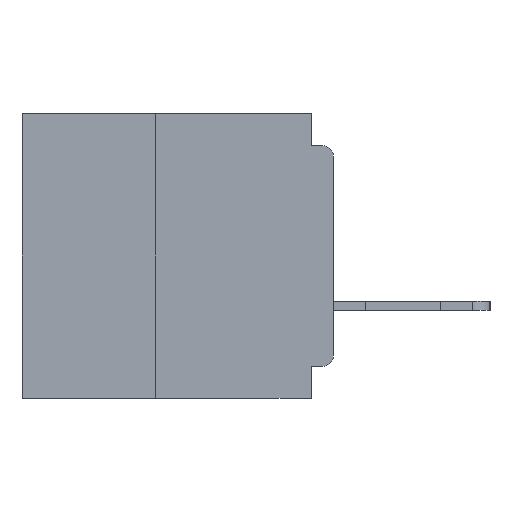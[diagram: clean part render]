
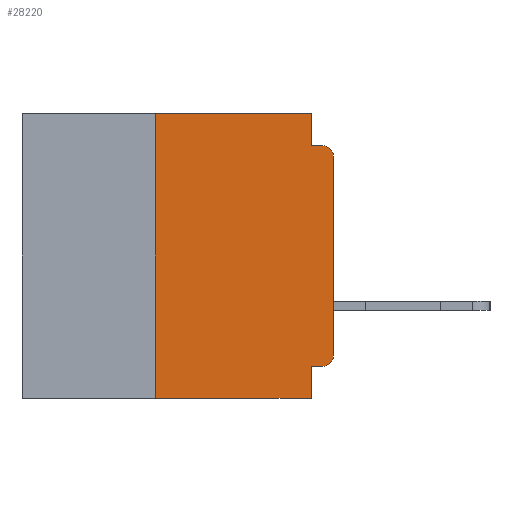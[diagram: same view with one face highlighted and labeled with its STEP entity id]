
A CAD part, left-side view. The second image highlights one B-rep face of the part: STEP entity #28220.
In plain terms, the highlighted planar face has unit normal (-1, 0, 0).
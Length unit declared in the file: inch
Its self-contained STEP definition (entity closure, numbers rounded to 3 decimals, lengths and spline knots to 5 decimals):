
#551 = EDGE_CURVE ( 'NONE', #10489, #44037, #18944, .T. ) ;
#1031 = DIRECTION ( 'NONE',  ( 0., -1., 0. ) ) ;
#2178 = DIRECTION ( 'NONE',  ( 0., 1., 0. ) ) ;
#2292 = VERTEX_POINT ( 'NONE', #49370 ) ;
#2967 = EDGE_LOOP ( 'NONE', ( #31060, #12646, #18318, #29580, #43339, #8762, #25555, #10824, #7437, #35365 ) ) ;
#3604 = EDGE_CURVE ( 'NONE', #47530, #10489, #49947, .T. ) ;
#5434 = DIRECTION ( 'NONE',  ( -1., 0., 0. ) ) ;
#6351 = CARTESIAN_POINT ( 'NONE',  ( 0., 0.031, 0. ) ) ;
#6486 = PLANE ( 'NONE',  #37413 ) ;
#6631 = CARTESIAN_POINT ( 'NONE',  ( 0., 0.015, -0.06 ) ) ;
#7437 = ORIENTED_EDGE ( 'NONE', *, *, #3604, .F. ) ;
#7501 = DIRECTION ( 'NONE',  ( 0., 0., 1. ) ) ;
#8411 = VECTOR ( 'NONE', #37831, 39.37008 ) ;
#8762 = ORIENTED_EDGE ( 'NONE', *, *, #16524, .F. ) ;
#9083 = VERTEX_POINT ( 'NONE', #19296 ) ;
#9841 = CARTESIAN_POINT ( 'NONE',  ( 0., 0.25, 0. ) ) ;
#9969 = VECTOR ( 'NONE', #1031, 39.37008 ) ;
#9994 = CARTESIAN_POINT ( 'NONE',  ( 0., 0.031, -0.045 ) ) ;
#10489 = VERTEX_POINT ( 'NONE', #37641 ) ;
#10625 = DIRECTION ( 'NONE',  ( 0., 0., -1. ) ) ;
#10824 = ORIENTED_EDGE ( 'NONE', *, *, #551, .F. ) ;
#11231 = EDGE_CURVE ( 'NONE', #26045, #44037, #18113, .T. ) ;
#11704 = VERTEX_POINT ( 'NONE', #6351 ) ;
#12646 = ORIENTED_EDGE ( 'NONE', *, *, #50050, .T. ) ;
#13008 = VECTOR ( 'NONE', #33981, 39.37008 ) ;
#13076 = CARTESIAN_POINT ( 'NONE',  ( 0., 0.015, -0.045 ) ) ;
#16524 = EDGE_CURVE ( 'NONE', #26045, #30975, #22703, .T. ) ;
#16795 = VECTOR ( 'NONE', #2178, 39.37008 ) ;
#16858 = VECTOR ( 'NONE', #22351, 39.37008 ) ;
#16990 = CARTESIAN_POINT ( 'NONE',  ( 0., 0.437, 0. ) ) ;
#17620 = CIRCLE ( 'NONE', #47769, 0.015 ) ;
#18113 = LINE ( 'NONE', #30441, #16858 ) ;
#18318 = ORIENTED_EDGE ( 'NONE', *, *, #27607, .F. ) ;
#18621 = DIRECTION ( 'NONE',  ( 1., 0., 0. ) ) ;
#18944 = LINE ( 'NONE', #34521, #8411 ) ;
#19296 = CARTESIAN_POINT ( 'NONE',  ( 0., 0., -0.34 ) ) ;
#22351 = DIRECTION ( 'NONE',  ( 0., -1., 0. ) ) ;
#22677 = DIRECTION ( 'NONE',  ( 0., -1., 0. ) ) ;
#22703 = LINE ( 'NONE', #27320, #40172 ) ;
#24415 = CARTESIAN_POINT ( 'NONE',  ( 0., 0.25, -0.4 ) ) ;
#24534 = EDGE_CURVE ( 'NONE', #11704, #38012, #26411, .T. ) ;
#25160 = VECTOR ( 'NONE', #31084, 39.37008 ) ;
#25555 = ORIENTED_EDGE ( 'NONE', *, *, #11231, .T. ) ;
#26045 = VERTEX_POINT ( 'NONE', #24415 ) ;
#26411 = LINE ( 'NONE', #27033, #25160 ) ;
#27033 = CARTESIAN_POINT ( 'NONE',  ( 0., 0.031, 0. ) ) ;
#27320 = CARTESIAN_POINT ( 'NONE',  ( 0., 0.25, -0.4 ) ) ;
#27607 = EDGE_CURVE ( 'NONE', #38012, #38303, #41369, .T. ) ;
#28220 = ADVANCED_FACE ( 'NONE', ( #32612 ), #6486, .F. ) ;
#29279 = CARTESIAN_POINT ( 'NONE',  ( 0., 0.015, -0.34 ) ) ;
#29580 = ORIENTED_EDGE ( 'NONE', *, *, #24534, .F. ) ;
#29904 = LINE ( 'NONE', #16990, #9969 ) ;
#30441 = CARTESIAN_POINT ( 'NONE',  ( 0., 0.437, -0.4 ) ) ;
#30975 = VERTEX_POINT ( 'NONE', #9841 ) ;
#31060 = ORIENTED_EDGE ( 'NONE', *, *, #51735, .T. ) ;
#31084 = DIRECTION ( 'NONE',  ( 0., 0., -1. ) ) ;
#32612 = FACE_OUTER_BOUND ( 'NONE', #2967, .T. ) ;
#33288 = DIRECTION ( 'NONE',  ( 0., 0., -1. ) ) ;
#33981 = DIRECTION ( 'NONE',  ( 0., 0., 1. ) ) ;
#34486 = DIRECTION ( 'NONE',  ( -1., 0., 0. ) ) ;
#34521 = CARTESIAN_POINT ( 'NONE',  ( 0., 0.031, -0.4 ) ) ;
#35365 = ORIENTED_EDGE ( 'NONE', *, *, #36639, .T. ) ;
#35439 = LINE ( 'NONE', #46005, #13008 ) ;
#36639 = EDGE_CURVE ( 'NONE', #47530, #9083, #17620, .T. ) ;
#37413 = AXIS2_PLACEMENT_3D ( 'NONE', #42325, #18621, #46559 ) ;
#37483 = CARTESIAN_POINT ( 'NONE',  ( 0., 0.031, -0.4 ) ) ;
#37641 = CARTESIAN_POINT ( 'NONE',  ( 0., 0.031, -0.355 ) ) ;
#37831 = DIRECTION ( 'NONE',  ( 0., 0., -1. ) ) ;
#38012 = VERTEX_POINT ( 'NONE', #9994 ) ;
#38303 = VERTEX_POINT ( 'NONE', #13076 ) ;
#40111 = VECTOR ( 'NONE', #22677, 39.37008 ) ;
#40172 = VECTOR ( 'NONE', #7501, 39.37008 ) ;
#41204 = CIRCLE ( 'NONE', #48235, 0.015 ) ;
#41369 = LINE ( 'NONE', #46622, #40111 ) ;
#42165 = EDGE_CURVE ( 'NONE', #30975, #11704, #29904, .T. ) ;
#42325 = CARTESIAN_POINT ( 'NONE',  ( 0., 0.437, 0. ) ) ;
#43339 = ORIENTED_EDGE ( 'NONE', *, *, #42165, .F. ) ;
#44037 = VERTEX_POINT ( 'NONE', #37483 ) ;
#46005 = CARTESIAN_POINT ( 'NONE',  ( 0., 0., 0. ) ) ;
#46559 = DIRECTION ( 'NONE',  ( 0., 0., -1. ) ) ;
#46622 = CARTESIAN_POINT ( 'NONE',  ( 0., 0., -0.045 ) ) ;
#47530 = VERTEX_POINT ( 'NONE', #51552 ) ;
#47769 = AXIS2_PLACEMENT_3D ( 'NONE', #29279, #5434, #33288 ) ;
#48235 = AXIS2_PLACEMENT_3D ( 'NONE', #6631, #34486, #10625 ) ;
#49370 = CARTESIAN_POINT ( 'NONE',  ( 0., 0., -0.06 ) ) ;
#49936 = CARTESIAN_POINT ( 'NONE',  ( 0., 0., -0.355 ) ) ;
#49947 = LINE ( 'NONE', #49936, #16795 ) ;
#50050 = EDGE_CURVE ( 'NONE', #2292, #38303, #41204, .T. ) ;
#51552 = CARTESIAN_POINT ( 'NONE',  ( 0., 0.015, -0.355 ) ) ;
#51735 = EDGE_CURVE ( 'NONE', #9083, #2292, #35439, .T. ) ;
